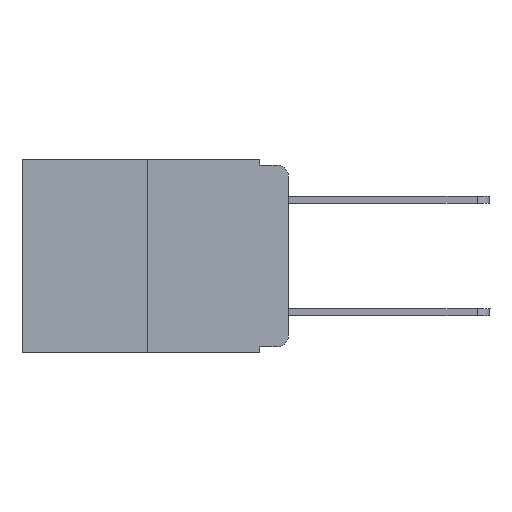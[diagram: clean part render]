
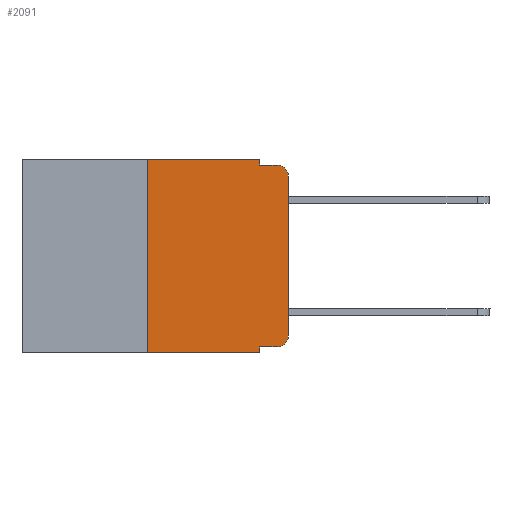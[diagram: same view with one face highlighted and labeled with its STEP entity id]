
A CAD part, left-side view. The second image highlights one B-rep face of the part: STEP entity #2091.
In plain terms, the highlighted planar face has unit normal (-1, 0, 0).
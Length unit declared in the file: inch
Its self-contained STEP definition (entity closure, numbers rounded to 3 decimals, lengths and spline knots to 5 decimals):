
#55 = EDGE_CURVE ( 'NONE', #3088, #2449, #6725, .T. ) ;
#177 = DIRECTION ( 'NONE',  ( 0., 0., -1. ) ) ;
#277 = VERTEX_POINT ( 'NONE', #6298 ) ;
#674 = VERTEX_POINT ( 'NONE', #2652 ) ;
#1038 = CARTESIAN_POINT ( 'NONE',  ( 0., 0.051, -0.333 ) ) ;
#1207 = VERTEX_POINT ( 'NONE', #1038 ) ;
#1323 = DIRECTION ( 'NONE',  ( 0., 0., -1. ) ) ;
#1432 = EDGE_CURVE ( 'NONE', #14077, #2449, #15083, .T. ) ;
#1486 = EDGE_LOOP ( 'NONE', ( #4110, #13253, #15565, #6115, #8623, #8209, #9344, #4059, #14087, #5109 ) ) ;
#1523 = EDGE_CURVE ( 'NONE', #1207, #4190, #13637, .T. ) ;
#1558 = CIRCLE ( 'NONE', #11047, 0.02 ) ;
#1923 = DIRECTION ( 'NONE',  ( 0., 0., -1. ) ) ;
#1936 = DIRECTION ( 'NONE',  ( -1., 0., 0. ) ) ;
#2091 = ADVANCED_FACE ( 'NONE', ( #12732 ), #13963, .F. ) ;
#2291 = LINE ( 'NONE', #4509, #11337 ) ;
#2449 = VERTEX_POINT ( 'NONE', #12623 ) ;
#2652 = CARTESIAN_POINT ( 'NONE',  ( 0., 0.051, 0. ) ) ;
#2962 = CARTESIAN_POINT ( 'NONE',  ( 0., 0.051, -0.333 ) ) ;
#3016 = VERTEX_POINT ( 'NONE', #11587 ) ;
#3088 = VERTEX_POINT ( 'NONE', #10601 ) ;
#3316 = CARTESIAN_POINT ( 'NONE',  ( 0., 0.25, 0. ) ) ;
#3813 = DIRECTION ( 'NONE',  ( 1., 0., 0. ) ) ;
#4059 = ORIENTED_EDGE ( 'NONE', *, *, #1523, .F. ) ;
#4081 = CARTESIAN_POINT ( 'NONE',  ( 0., 0.051, -0.01 ) ) ;
#4110 = ORIENTED_EDGE ( 'NONE', *, *, #5791, .T. ) ;
#4153 = VECTOR ( 'NONE', #8897, 39.37008 ) ;
#4190 = VERTEX_POINT ( 'NONE', #14835 ) ;
#4433 = DIRECTION ( 'NONE',  ( 0., -1., 0. ) ) ;
#4465 = VECTOR ( 'NONE', #5855, 39.37008 ) ;
#4509 = CARTESIAN_POINT ( 'NONE',  ( 0., 0.473, 0. ) ) ;
#5109 = ORIENTED_EDGE ( 'NONE', *, *, #15891, .T. ) ;
#5283 = CARTESIAN_POINT ( 'NONE',  ( 0., 0.02, -0.313 ) ) ;
#5406 = LINE ( 'NONE', #2962, #8278 ) ;
#5633 = CARTESIAN_POINT ( 'NONE',  ( 0., 0.051, 0. ) ) ;
#5791 = EDGE_CURVE ( 'NONE', #11170, #14077, #14925, .T. ) ;
#5855 = DIRECTION ( 'NONE',  ( 0., 0., 1. ) ) ;
#6115 = ORIENTED_EDGE ( 'NONE', *, *, #11590, .F. ) ;
#6143 = DIRECTION ( 'NONE',  ( 0., 0., -1. ) ) ;
#6298 = CARTESIAN_POINT ( 'NONE',  ( 0., 0.25, -0.343 ) ) ;
#6337 = LINE ( 'NONE', #10132, #4153 ) ;
#6647 = EDGE_CURVE ( 'NONE', #1207, #3016, #5406, .T. ) ;
#6725 = LINE ( 'NONE', #4081, #11357 ) ;
#7563 = VERTEX_POINT ( 'NONE', #3316 ) ;
#8045 = LINE ( 'NONE', #5633, #11445 ) ;
#8209 = ORIENTED_EDGE ( 'NONE', *, *, #9772, .F. ) ;
#8278 = VECTOR ( 'NONE', #15408, 39.37008 ) ;
#8623 = ORIENTED_EDGE ( 'NONE', *, *, #14917, .F. ) ;
#8686 = VECTOR ( 'NONE', #4433, 39.37008 ) ;
#8897 = DIRECTION ( 'NONE',  ( 0., 0., 1. ) ) ;
#9344 = ORIENTED_EDGE ( 'NONE', *, *, #13781, .T. ) ;
#9563 = AXIS2_PLACEMENT_3D ( 'NONE', #15204, #3813, #177 ) ;
#9615 = DIRECTION ( 'NONE',  ( 0., -1., 0. ) ) ;
#9772 = EDGE_CURVE ( 'NONE', #277, #7563, #6337, .T. ) ;
#10132 = CARTESIAN_POINT ( 'NONE',  ( 0., 0.25, 0. ) ) ;
#10469 = CARTESIAN_POINT ( 'NONE',  ( 0., 0.473, -0.343 ) ) ;
#10601 = CARTESIAN_POINT ( 'NONE',  ( 0., 0.051, -0.01 ) ) ;
#10712 = LINE ( 'NONE', #10469, #8686 ) ;
#11047 = AXIS2_PLACEMENT_3D ( 'NONE', #5283, #12953, #1323 ) ;
#11170 = VERTEX_POINT ( 'NONE', #11625 ) ;
#11337 = VECTOR ( 'NONE', #9615, 39.37008 ) ;
#11357 = VECTOR ( 'NONE', #14149, 39.37008 ) ;
#11445 = VECTOR ( 'NONE', #1923, 39.37008 ) ;
#11587 = CARTESIAN_POINT ( 'NONE',  ( 0., 0.02, -0.333 ) ) ;
#11590 = EDGE_CURVE ( 'NONE', #674, #3088, #8045, .T. ) ;
#11625 = CARTESIAN_POINT ( 'NONE',  ( 0., 0., -0.313 ) ) ;
#11662 = AXIS2_PLACEMENT_3D ( 'NONE', #12080, #1936, #15795 ) ;
#12080 = CARTESIAN_POINT ( 'NONE',  ( 0., 0.02, -0.03 ) ) ;
#12623 = CARTESIAN_POINT ( 'NONE',  ( 0., 0.02, -0.01 ) ) ;
#12732 = FACE_OUTER_BOUND ( 'NONE', #1486, .T. ) ;
#12882 = CARTESIAN_POINT ( 'NONE',  ( 0., 0., -0.03 ) ) ;
#12953 = DIRECTION ( 'NONE',  ( -1., 0., 0. ) ) ;
#13253 = ORIENTED_EDGE ( 'NONE', *, *, #1432, .T. ) ;
#13637 = LINE ( 'NONE', #16203, #15612 ) ;
#13781 = EDGE_CURVE ( 'NONE', #277, #4190, #10712, .T. ) ;
#13963 = PLANE ( 'NONE',  #9563 ) ;
#14077 = VERTEX_POINT ( 'NONE', #12882 ) ;
#14087 = ORIENTED_EDGE ( 'NONE', *, *, #6647, .T. ) ;
#14149 = DIRECTION ( 'NONE',  ( 0., -1., 0. ) ) ;
#14835 = CARTESIAN_POINT ( 'NONE',  ( 0., 0.051, -0.343 ) ) ;
#14917 = EDGE_CURVE ( 'NONE', #7563, #674, #2291, .T. ) ;
#14925 = LINE ( 'NONE', #16167, #4465 ) ;
#15083 = CIRCLE ( 'NONE', #11662, 0.02 ) ;
#15204 = CARTESIAN_POINT ( 'NONE',  ( 0., 0.473, 0. ) ) ;
#15408 = DIRECTION ( 'NONE',  ( 0., -1., 0. ) ) ;
#15565 = ORIENTED_EDGE ( 'NONE', *, *, #55, .F. ) ;
#15612 = VECTOR ( 'NONE', #6143, 39.37008 ) ;
#15795 = DIRECTION ( 'NONE',  ( 0., 0., -1. ) ) ;
#15891 = EDGE_CURVE ( 'NONE', #3016, #11170, #1558, .T. ) ;
#16167 = CARTESIAN_POINT ( 'NONE',  ( 0., 0., 0. ) ) ;
#16203 = CARTESIAN_POINT ( 'NONE',  ( 0., 0.051, 0. ) ) ;
